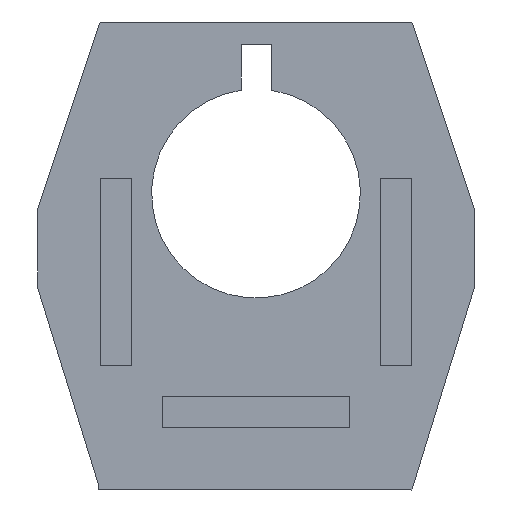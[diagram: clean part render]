
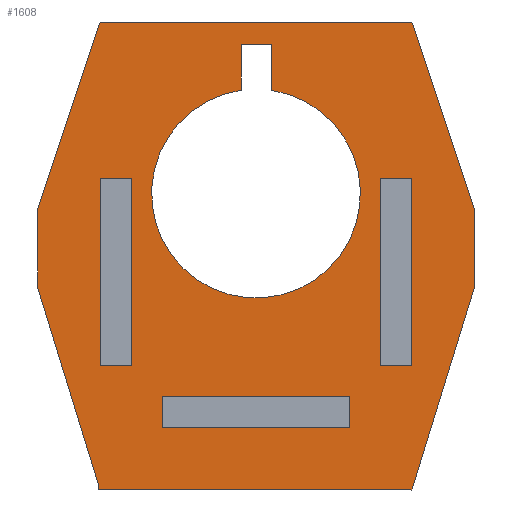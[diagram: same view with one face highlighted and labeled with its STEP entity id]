
A CAD part, front view. The second image highlights one B-rep face of the part: STEP entity #1608.
In plain terms, the highlighted planar face has unit normal (0, -1, 0).
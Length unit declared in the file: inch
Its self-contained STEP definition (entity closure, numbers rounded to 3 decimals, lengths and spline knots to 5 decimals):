
#20=CIRCLE('',#1694,0.33465);
#27=FACE_BOUND('',#181,.T.);
#28=FACE_BOUND('',#182,.T.);
#29=FACE_BOUND('',#183,.T.);
#30=FACE_BOUND('',#184,.T.);
#92=FACE_OUTER_BOUND('',#180,.T.);
#180=EDGE_LOOP('',(#1284,#1285,#1286,#1287,#1288,#1289,#1290,#1291,#1292));
#181=EDGE_LOOP('',(#1293,#1294,#1295,#1296));
#182=EDGE_LOOP('',(#1297,#1298,#1299,#1300));
#183=EDGE_LOOP('',(#1301,#1302,#1303,#1304));
#184=EDGE_LOOP('',(#1305,#1306,#1307,#1308));
#291=LINE('',#2281,#509);
#294=LINE('',#2286,#512);
#302=LINE('',#2304,#520);
#306=LINE('',#2311,#524);
#309=LINE('',#2317,#527);
#315=LINE('',#2331,#533);
#318=LINE('',#2336,#536);
#334=LINE('',#2372,#552);
#337=LINE('',#2377,#555);
#339=LINE('',#2381,#557);
#342=LINE('',#2387,#560);
#343=LINE('',#2390,#561);
#345=LINE('',#2393,#563);
#346=LINE('',#2396,#564);
#348=LINE('',#2399,#566);
#349=LINE('',#2403,#567);
#352=LINE('',#2408,#570);
#354=LINE('',#2412,#572);
#356=LINE('',#2416,#574);
#358=LINE('',#2420,#576);
#360=LINE('',#2424,#578);
#362=LINE('',#2428,#580);
#364=LINE('',#2432,#582);
#366=LINE('',#2435,#584);
#509=VECTOR('',#1858,0.3937);
#512=VECTOR('',#1863,0.3937);
#520=VECTOR('',#1879,0.3937);
#524=VECTOR('',#1885,0.3937);
#527=VECTOR('',#1890,0.3937);
#533=VECTOR('',#1900,0.3937);
#536=VECTOR('',#1905,0.3937);
#552=VECTOR('',#1929,0.3937);
#555=VECTOR('',#1934,0.3937);
#557=VECTOR('',#1938,0.3937);
#560=VECTOR('',#1947,0.3937);
#561=VECTOR('',#1950,0.3937);
#563=VECTOR('',#1954,0.3937);
#564=VECTOR('',#1957,0.3937);
#566=VECTOR('',#1961,0.3937);
#567=VECTOR('',#1964,0.3937);
#570=VECTOR('',#1969,0.3937);
#572=VECTOR('',#1973,0.3937);
#574=VECTOR('',#1977,0.3937);
#576=VECTOR('',#1981,0.3937);
#578=VECTOR('',#1985,0.3937);
#580=VECTOR('',#1989,0.3937);
#582=VECTOR('',#1993,0.3937);
#584=VECTOR('',#1997,0.3937);
#708=VERTEX_POINT('',#2278);
#709=VERTEX_POINT('',#2280);
#710=VERTEX_POINT('',#2284);
#715=VERTEX_POINT('',#2301);
#716=VERTEX_POINT('',#2303);
#718=VERTEX_POINT('',#2309);
#720=VERTEX_POINT('',#2315);
#725=VERTEX_POINT('',#2328);
#726=VERTEX_POINT('',#2330);
#727=VERTEX_POINT('',#2334);
#742=VERTEX_POINT('',#2370);
#743=VERTEX_POINT('',#2371);
#744=VERTEX_POINT('',#2376);
#745=VERTEX_POINT('',#2380);
#746=VERTEX_POINT('',#2389);
#747=VERTEX_POINT('',#2395);
#748=VERTEX_POINT('',#2401);
#749=VERTEX_POINT('',#2402);
#750=VERTEX_POINT('',#2407);
#751=VERTEX_POINT('',#2411);
#752=VERTEX_POINT('',#2415);
#753=VERTEX_POINT('',#2419);
#754=VERTEX_POINT('',#2423);
#755=VERTEX_POINT('',#2427);
#756=VERTEX_POINT('',#2431);
#875=EDGE_CURVE('',#708,#709,#291,.T.);
#878=EDGE_CURVE('',#710,#708,#294,.T.);
#886=EDGE_CURVE('',#715,#716,#302,.T.);
#890=EDGE_CURVE('',#718,#715,#306,.T.);
#893=EDGE_CURVE('',#720,#718,#309,.T.);
#899=EDGE_CURVE('',#725,#726,#315,.T.);
#902=EDGE_CURVE('',#727,#725,#318,.T.);
#919=EDGE_CURVE('',#742,#743,#334,.T.);
#922=EDGE_CURVE('',#743,#744,#337,.T.);
#924=EDGE_CURVE('',#744,#745,#339,.T.);
#926=EDGE_CURVE('',#745,#742,#20,.T.);
#928=EDGE_CURVE('',#716,#720,#342,.T.);
#929=EDGE_CURVE('',#726,#746,#343,.T.);
#931=EDGE_CURVE('',#746,#727,#345,.T.);
#932=EDGE_CURVE('',#709,#747,#346,.T.);
#934=EDGE_CURVE('',#747,#710,#348,.T.);
#935=EDGE_CURVE('',#748,#749,#349,.T.);
#938=EDGE_CURVE('',#749,#750,#352,.T.);
#940=EDGE_CURVE('',#750,#751,#354,.T.);
#942=EDGE_CURVE('',#751,#752,#356,.T.);
#944=EDGE_CURVE('',#752,#753,#358,.T.);
#946=EDGE_CURVE('',#753,#754,#360,.T.);
#948=EDGE_CURVE('',#754,#755,#362,.T.);
#950=EDGE_CURVE('',#755,#756,#364,.T.);
#952=EDGE_CURVE('',#756,#748,#366,.T.);
#1284=ORIENTED_EDGE('',*,*,#952,.T.);
#1285=ORIENTED_EDGE('',*,*,#935,.T.);
#1286=ORIENTED_EDGE('',*,*,#938,.T.);
#1287=ORIENTED_EDGE('',*,*,#940,.T.);
#1288=ORIENTED_EDGE('',*,*,#942,.T.);
#1289=ORIENTED_EDGE('',*,*,#944,.T.);
#1290=ORIENTED_EDGE('',*,*,#946,.T.);
#1291=ORIENTED_EDGE('',*,*,#948,.T.);
#1292=ORIENTED_EDGE('',*,*,#950,.T.);
#1293=ORIENTED_EDGE('',*,*,#934,.F.);
#1294=ORIENTED_EDGE('',*,*,#932,.F.);
#1295=ORIENTED_EDGE('',*,*,#875,.F.);
#1296=ORIENTED_EDGE('',*,*,#878,.F.);
#1297=ORIENTED_EDGE('',*,*,#931,.F.);
#1298=ORIENTED_EDGE('',*,*,#929,.F.);
#1299=ORIENTED_EDGE('',*,*,#899,.F.);
#1300=ORIENTED_EDGE('',*,*,#902,.F.);
#1301=ORIENTED_EDGE('',*,*,#893,.F.);
#1302=ORIENTED_EDGE('',*,*,#928,.F.);
#1303=ORIENTED_EDGE('',*,*,#886,.F.);
#1304=ORIENTED_EDGE('',*,*,#890,.F.);
#1305=ORIENTED_EDGE('',*,*,#926,.T.);
#1306=ORIENTED_EDGE('',*,*,#919,.T.);
#1307=ORIENTED_EDGE('',*,*,#922,.T.);
#1308=ORIENTED_EDGE('',*,*,#924,.T.);
#1525=PLANE('',#1709);
#1608=ADVANCED_FACE('',(#92,#27,#28,#29,#30),#1525,.F.);
#1694=AXIS2_PLACEMENT_3D('',#2384,#1942,#1943);
#1709=AXIS2_PLACEMENT_3D('',#2436,#1998,#1999);
#1858=DIRECTION('',(0.,0.,-1.));
#1863=DIRECTION('',(-1.,0.,0.));
#1879=DIRECTION('',(0.,0.,-1.));
#1885=DIRECTION('',(-1.,0.,0.));
#1890=DIRECTION('',(0.,0.,1.));
#1900=DIRECTION('',(0.,0.,-1.));
#1905=DIRECTION('',(-1.,0.,0.));
#1929=DIRECTION('',(0.,0.,1.));
#1934=DIRECTION('',(1.,0.,0.));
#1938=DIRECTION('',(0.,0.,-1.));
#1942=DIRECTION('center_axis',(0.,1.,0.));
#1943=DIRECTION('ref_axis',(-1.,0.,0.));
#1947=DIRECTION('',(1.,0.,0.));
#1950=DIRECTION('',(1.,0.,0.));
#1954=DIRECTION('',(0.,0.,1.));
#1957=DIRECTION('',(1.,0.,0.));
#1961=DIRECTION('',(0.,0.,1.));
#1964=DIRECTION('',(0.,0.,-1.));
#1969=DIRECTION('',(1.,0.,0.));
#1973=DIRECTION('',(0.294,0.,0.956));
#1977=DIRECTION('',(0.,0.,1.));
#1981=DIRECTION('',(-0.316,0.,0.949));
#1985=DIRECTION('',(-1.,0.,0.));
#1989=DIRECTION('',(-0.316,0.,-0.949));
#1993=DIRECTION('',(0.,0.,-1.));
#1997=DIRECTION('',(0.294,0.,-0.956));
#1998=DIRECTION('center_axis',(0.,1.,0.));
#1999=DIRECTION('ref_axis',(-1.,0.,0.));
#2278=CARTESIAN_POINT('',(-0.5,7.6,0.5));
#2280=CARTESIAN_POINT('',(-0.5,7.6,-0.1));
#2281=CARTESIAN_POINT('',(-0.5,7.6,0.075));
#2284=CARTESIAN_POINT('',(-0.4,7.6,0.5));
#2286=CARTESIAN_POINT('',(-0.25,7.6,0.5));
#2301=CARTESIAN_POINT('',(0.4,7.6,0.5));
#2303=CARTESIAN_POINT('',(0.4,7.6,-0.1));
#2304=CARTESIAN_POINT('',(0.4,7.6,0.075));
#2309=CARTESIAN_POINT('',(0.5,7.6,0.5));
#2311=CARTESIAN_POINT('',(0.2,7.6,0.5));
#2315=CARTESIAN_POINT('',(0.5,7.6,-0.1));
#2317=CARTESIAN_POINT('',(0.5,7.6,0.375));
#2328=CARTESIAN_POINT('',(-0.3,7.6,-0.2));
#2330=CARTESIAN_POINT('',(-0.3,7.6,-0.3));
#2331=CARTESIAN_POINT('',(-0.3,7.6,-0.025));
#2334=CARTESIAN_POINT('',(0.3,7.6,-0.2));
#2336=CARTESIAN_POINT('',(-0.15,7.6,-0.2));
#2370=CARTESIAN_POINT('',(-0.0477,7.6,0.78123));
#2371=CARTESIAN_POINT('',(-0.0477,7.6,0.92834));
#2372=CARTESIAN_POINT('',(-0.0477,7.6,0.58917));
#2376=CARTESIAN_POINT('',(0.05072,7.6,0.92834));
#2377=CARTESIAN_POINT('',(0.02536,7.6,0.92834));
#2380=CARTESIAN_POINT('',(0.05072,7.6,0.78078));
#2381=CARTESIAN_POINT('',(0.05072,7.6,0.51539));
#2384=CARTESIAN_POINT('Origin',(0.,7.6,0.45));
#2387=CARTESIAN_POINT('',(0.25,7.6,-0.1));
#2389=CARTESIAN_POINT('',(0.3,7.6,-0.3));
#2390=CARTESIAN_POINT('',(0.15,7.6,-0.3));
#2393=CARTESIAN_POINT('',(0.3,7.6,0.025));
#2395=CARTESIAN_POINT('',(-0.4,7.6,-0.1));
#2396=CARTESIAN_POINT('',(-0.2,7.6,-0.1));
#2399=CARTESIAN_POINT('',(-0.4,7.6,0.375));
#2401=CARTESIAN_POINT('',(-0.50506,7.6,-0.48354));
#2402=CARTESIAN_POINT('',(-0.50506,7.6,-0.5));
#2403=CARTESIAN_POINT('',(-0.50506,7.6,0.625));
#2407=CARTESIAN_POINT('',(0.5,7.6,-0.5));
#2408=CARTESIAN_POINT('',(-0.2,7.6,-0.5));
#2411=CARTESIAN_POINT('',(0.7,7.6,0.15));
#2412=CARTESIAN_POINT('',(0.68378,7.6,0.0973));
#2415=CARTESIAN_POINT('',(0.7,7.6,0.4));
#2416=CARTESIAN_POINT('',(0.7,7.6,0.325));
#2419=CARTESIAN_POINT('',(0.5,7.6,1.));
#2420=CARTESIAN_POINT('',(0.5875,7.6,0.7375));
#2423=CARTESIAN_POINT('',(-0.5,7.6,1.));
#2424=CARTESIAN_POINT('',(-0.25,7.6,1.));
#2427=CARTESIAN_POINT('',(-0.7,7.6,0.4));
#2428=CARTESIAN_POINT('',(-0.6875,7.6,0.4375));
#2431=CARTESIAN_POINT('',(-0.7,7.6,0.15));
#2432=CARTESIAN_POINT('',(-0.7,7.6,0.2));
#2435=CARTESIAN_POINT('',(-0.58378,7.6,-0.2277));
#2436=CARTESIAN_POINT('Origin',(0.,7.6,0.25));
